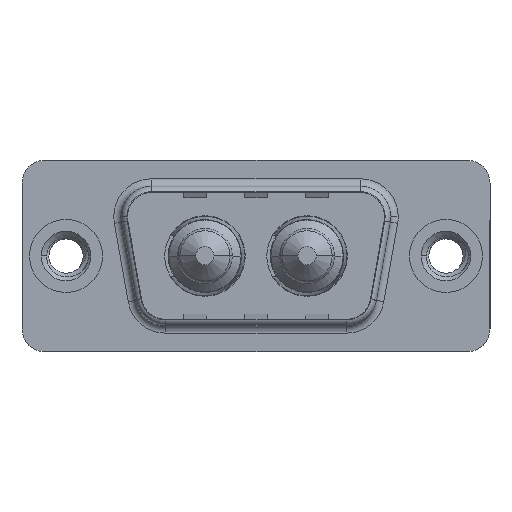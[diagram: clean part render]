
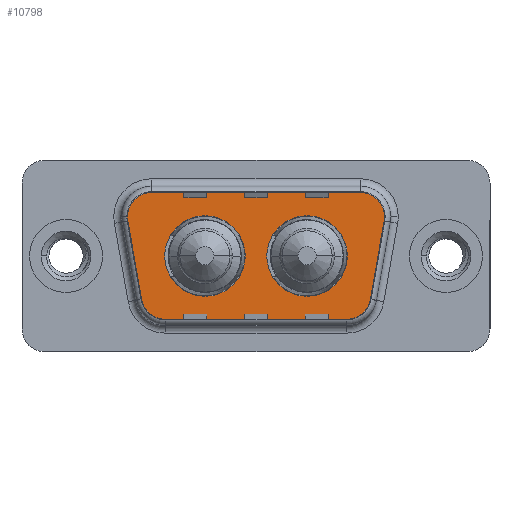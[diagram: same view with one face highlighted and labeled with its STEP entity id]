
A CAD part, top view. The second image highlights one B-rep face of the part: STEP entity #10798.
In plain terms, the highlighted planar face has unit normal (0, 0, 1).
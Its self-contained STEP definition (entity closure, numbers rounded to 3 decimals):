
#27 = DIRECTION ( 'NONE',  ( 0., 0., 1. ) ) ;
#127 = CARTESIAN_POINT ( 'NONE',  ( 5.436, 2.9, 0. ) ) ;
#162 = VERTEX_POINT ( 'NONE', #10662 ) ;
#251 = EDGE_CURVE ( 'NONE', #1419, #945, #4740, .T. ) ;
#314 = EDGE_CURVE ( 'NONE', #1428, #1059, #3922, .T. ) ;
#375 = VERTEX_POINT ( 'NONE', #1781 ) ;
#541 = DIRECTION ( 'NONE',  ( 1., 0., 0. ) ) ;
#543 = CARTESIAN_POINT ( 'NONE',  ( 5.436, 4.9, 0. ) ) ;
#676 = CARTESIAN_POINT ( 'NONE',  ( 18.541, -4.9, 0. ) ) ;
#945 = VERTEX_POINT ( 'NONE', #4898 ) ;
#1026 = DIRECTION ( 'NONE',  ( 1., 0., 0. ) ) ;
#1059 = VERTEX_POINT ( 'NONE', #4537 ) ;
#1060 = AXIS2_PLACEMENT_3D ( 'NONE', #127, #6313, #1026 ) ;
#1096 = VECTOR ( 'NONE', #6099, 1000. ) ;
#1227 = EDGE_CURVE ( 'NONE', #1059, #162, #5552, .T. ) ;
#1245 = EDGE_CURVE ( 'NONE', #9416, #2015, #3492, .T. ) ;
#1286 = DIRECTION ( 'NONE',  ( 0., 0., 1. ) ) ;
#1419 = VERTEX_POINT ( 'NONE', #1529 ) ;
#1428 = VERTEX_POINT ( 'NONE', #8330 ) ;
#1445 = ORIENTED_EDGE ( 'NONE', *, *, #10002, .F. ) ;
#1529 = CARTESIAN_POINT ( 'NONE',  ( 11.79, 0., 0. ) ) ;
#1573 = AXIS2_PLACEMENT_3D ( 'NONE', #4065, #10309, #4944 ) ;
#1660 = CIRCLE ( 'NONE', #2533, 2. ) ;
#1781 = CARTESIAN_POINT ( 'NONE',  ( 18.51, 0., 0. ) ) ;
#1913 = CARTESIAN_POINT ( 'NONE',  ( 6.459, -4.9, 0. ) ) ;
#1922 = FACE_OUTER_BOUND ( 'NONE', #11365, .T. ) ;
#1981 = DIRECTION ( 'NONE',  ( 0., 0., 1. ) ) ;
#2015 = VERTEX_POINT ( 'NONE', #8069 ) ;
#2061 = CARTESIAN_POINT ( 'NONE',  ( 5.436, 4.9, 0. ) ) ;
#2090 = CARTESIAN_POINT ( 'NONE',  ( 13.21, 0., 0. ) ) ;
#2285 = CARTESIAN_POINT ( 'NONE',  ( 19.564, 2.9, 0. ) ) ;
#2354 = CARTESIAN_POINT ( 'NONE',  ( 3.466, 2.553, 0. ) ) ;
#2444 = DIRECTION ( 'NONE',  ( 0., 0., 1. ) ) ;
#2520 = DIRECTION ( 'NONE',  ( 1., 0., 0. ) ) ;
#2533 = AXIS2_PLACEMENT_3D ( 'NONE', #2285, #8525, #3167 ) ;
#2766 = VECTOR ( 'NONE', #10781, 1000. ) ;
#2849 = AXIS2_PLACEMENT_3D ( 'NONE', #9263, #3921, #6959 ) ;
#3011 = ORIENTED_EDGE ( 'NONE', *, *, #1245, .T. ) ;
#3013 = VERTEX_POINT ( 'NONE', #6657 ) ;
#3088 = AXIS2_PLACEMENT_3D ( 'NONE', #7975, #2444, #2520 ) ;
#3167 = DIRECTION ( 'NONE',  ( -1., 0., 0. ) ) ;
#3440 = LINE ( 'NONE', #11438, #1096 ) ;
#3492 = CIRCLE ( 'NONE', #4045, 2. ) ;
#3729 = VECTOR ( 'NONE', #6735, 1000. ) ;
#3797 = ORIENTED_EDGE ( 'NONE', *, *, #10327, .T. ) ;
#3921 = DIRECTION ( 'NONE',  ( 0., 0., 1. ) ) ;
#3922 = LINE ( 'NONE', #7407, #8671 ) ;
#4045 = AXIS2_PLACEMENT_3D ( 'NONE', #11390, #9573, #6364 ) ;
#4049 = PLANE ( 'NONE',  #5648 ) ;
#4062 = EDGE_CURVE ( 'NONE', #9859, #10380, #6225, .T. ) ;
#4065 = CARTESIAN_POINT ( 'NONE',  ( 9.14, 0., 0. ) ) ;
#4245 = VERTEX_POINT ( 'NONE', #2090 ) ;
#4537 = CARTESIAN_POINT ( 'NONE',  ( 21.534, 2.553, 0. ) ) ;
#4540 = FACE_BOUND ( 'NONE', #10466, .T. ) ;
#4642 = ORIENTED_EDGE ( 'NONE', *, *, #1227, .T. ) ;
#4740 = CIRCLE ( 'NONE', #3088, 2.65 ) ;
#4741 = AXIS2_PLACEMENT_3D ( 'NONE', #7282, #1981, #8208 ) ;
#4898 = CARTESIAN_POINT ( 'NONE',  ( 6.49, 0., 0. ) ) ;
#4944 = DIRECTION ( 'NONE',  ( 1., 0., 0. ) ) ;
#5032 = ORIENTED_EDGE ( 'NONE', *, *, #8358, .T. ) ;
#5108 = LINE ( 'NONE', #1913, #2766 ) ;
#5203 = EDGE_CURVE ( 'NONE', #375, #4245, #9044, .T. ) ;
#5304 = EDGE_CURVE ( 'NONE', #3013, #9859, #5824, .T. ) ;
#5307 = CARTESIAN_POINT ( 'NONE',  ( 18.541, -2.9, 0. ) ) ;
#5405 = ORIENTED_EDGE ( 'NONE', *, *, #5203, .F. ) ;
#5416 = CIRCLE ( 'NONE', #11461, 2. ) ;
#5552 = CIRCLE ( 'NONE', #2849, 2. ) ;
#5648 = AXIS2_PLACEMENT_3D ( 'NONE', #11170, #5836, #541 ) ;
#5657 = ORIENTED_EDGE ( 'NONE', *, *, #4062, .T. ) ;
#5718 = EDGE_CURVE ( 'NONE', #2015, #9476, #5108, .T. ) ;
#5824 = LINE ( 'NONE', #543, #3729 ) ;
#5836 = DIRECTION ( 'NONE',  ( 0., 0., 1. ) ) ;
#6097 = CIRCLE ( 'NONE', #4741, 2.65 ) ;
#6099 = DIRECTION ( 'NONE',  ( 0.174, -0.985, 0. ) ) ;
#6208 = DIRECTION ( 'NONE',  ( 1., 0., 0. ) ) ;
#6225 = CIRCLE ( 'NONE', #1060, 2. ) ;
#6313 = DIRECTION ( 'NONE',  ( 0., 0., 1. ) ) ;
#6364 = DIRECTION ( 'NONE',  ( -1., 0., 0. ) ) ;
#6580 = CARTESIAN_POINT ( 'NONE',  ( 15.86, 0., 0. ) ) ;
#6657 = CARTESIAN_POINT ( 'NONE',  ( 19.564, 4.9, 0. ) ) ;
#6735 = DIRECTION ( 'NONE',  ( -1., 0., 0. ) ) ;
#6839 = CARTESIAN_POINT ( 'NONE',  ( 4.489, -3.247, 0. ) ) ;
#6959 = DIRECTION ( 'NONE',  ( -1., 0., 0. ) ) ;
#7282 = CARTESIAN_POINT ( 'NONE',  ( 15.86, 0., 0. ) ) ;
#7407 = CARTESIAN_POINT ( 'NONE',  ( 21.534, 2.553, 0. ) ) ;
#7473 = DIRECTION ( 'NONE',  ( 1., 0., 0. ) ) ;
#7975 = CARTESIAN_POINT ( 'NONE',  ( 9.14, 0., 0. ) ) ;
#8069 = CARTESIAN_POINT ( 'NONE',  ( 6.459, -4.9, 0. ) ) ;
#8208 = DIRECTION ( 'NONE',  ( 1., 0., 0. ) ) ;
#8330 = CARTESIAN_POINT ( 'NONE',  ( 20.511, -3.247, 0. ) ) ;
#8358 = EDGE_CURVE ( 'NONE', #9476, #1428, #5416, .T. ) ;
#8436 = ORIENTED_EDGE ( 'NONE', *, *, #314, .T. ) ;
#8525 = DIRECTION ( 'NONE',  ( 0., 0., 1. ) ) ;
#8671 = VECTOR ( 'NONE', #9691, 1000. ) ;
#8909 = CIRCLE ( 'NONE', #1573, 2.65 ) ;
#9025 = FACE_BOUND ( 'NONE', #10048, .T. ) ;
#9044 = CIRCLE ( 'NONE', #10523, 2.65 ) ;
#9076 = ORIENTED_EDGE ( 'NONE', *, *, #251, .F. ) ;
#9263 = CARTESIAN_POINT ( 'NONE',  ( 19.564, 2.9, 0. ) ) ;
#9416 = VERTEX_POINT ( 'NONE', #6839 ) ;
#9476 = VERTEX_POINT ( 'NONE', #676 ) ;
#9573 = DIRECTION ( 'NONE',  ( 0., 0., 1. ) ) ;
#9691 = DIRECTION ( 'NONE',  ( 0.174, 0.985, 0. ) ) ;
#9772 = EDGE_CURVE ( 'NONE', #4245, #375, #6097, .T. ) ;
#9859 = VERTEX_POINT ( 'NONE', #2061 ) ;
#10002 = EDGE_CURVE ( 'NONE', #945, #1419, #8909, .T. ) ;
#10025 = ORIENTED_EDGE ( 'NONE', *, *, #5718, .T. ) ;
#10048 = EDGE_LOOP ( 'NONE', ( #5405, #11458 ) ) ;
#10284 = ORIENTED_EDGE ( 'NONE', *, *, #10912, .T. ) ;
#10309 = DIRECTION ( 'NONE',  ( 0., 0., 1. ) ) ;
#10327 = EDGE_CURVE ( 'NONE', #162, #3013, #1660, .T. ) ;
#10380 = VERTEX_POINT ( 'NONE', #2354 ) ;
#10466 = EDGE_LOOP ( 'NONE', ( #9076, #1445 ) ) ;
#10523 = AXIS2_PLACEMENT_3D ( 'NONE', #6580, #1286, #7473 ) ;
#10662 = CARTESIAN_POINT ( 'NONE',  ( 21.564, 2.9, 0. ) ) ;
#10781 = DIRECTION ( 'NONE',  ( 1., 0., 0. ) ) ;
#10798 = ADVANCED_FACE ( 'NONE', ( #9025, #4540, #1922 ), #4049, .T. ) ;
#10912 = EDGE_CURVE ( 'NONE', #10380, #9416, #3440, .T. ) ;
#11170 = CARTESIAN_POINT ( 'NONE',  ( 18.541, -2.9, 0. ) ) ;
#11336 = ORIENTED_EDGE ( 'NONE', *, *, #5304, .T. ) ;
#11365 = EDGE_LOOP ( 'NONE', ( #5032, #8436, #4642, #3797, #11336, #5657, #10284, #3011, #10025 ) ) ;
#11390 = CARTESIAN_POINT ( 'NONE',  ( 6.459, -2.9, 0. ) ) ;
#11438 = CARTESIAN_POINT ( 'NONE',  ( 3.466, 2.553, 0. ) ) ;
#11458 = ORIENTED_EDGE ( 'NONE', *, *, #9772, .F. ) ;
#11461 = AXIS2_PLACEMENT_3D ( 'NONE', #5307, #27, #6208 ) ;
